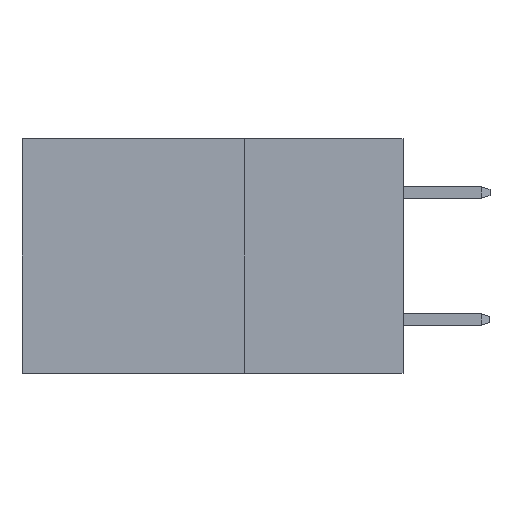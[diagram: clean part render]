
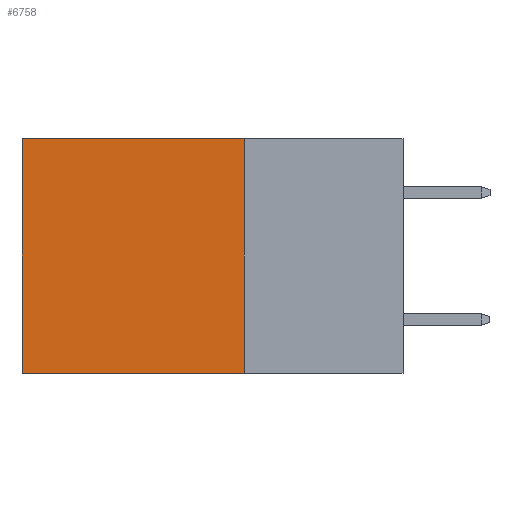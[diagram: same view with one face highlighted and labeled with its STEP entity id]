
A CAD part, left-side view. The second image highlights one B-rep face of the part: STEP entity #6758.
In plain terms, the highlighted planar face has unit normal (-1, 0, 0).
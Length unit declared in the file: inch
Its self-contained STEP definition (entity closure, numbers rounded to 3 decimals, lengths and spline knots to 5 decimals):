
#52 = VERTEX_POINT ( 'NONE', #12738 ) ;
#105 = CARTESIAN_POINT ( 'NONE',  ( 0.2875, 0.6, -0.37 ) ) ;
#437 = ORIENTED_EDGE ( 'NONE', *, *, #8776, .F. ) ;
#654 = DIRECTION ( 'NONE',  ( 0., 0., -1. ) ) ;
#732 = DIRECTION ( 'NONE',  ( 1., 0., 0. ) ) ;
#789 = EDGE_CURVE ( 'NONE', #52, #1972, #9901, .T. ) ;
#849 = PLANE ( 'NONE',  #10266 ) ;
#1972 = VERTEX_POINT ( 'NONE', #105 ) ;
#2182 = VERTEX_POINT ( 'NONE', #2674 ) ;
#2674 = CARTESIAN_POINT ( 'NONE',  ( 0.2875, 0.25, -0.37 ) ) ;
#2708 = ORIENTED_EDGE ( 'NONE', *, *, #7751, .T. ) ;
#2967 = CARTESIAN_POINT ( 'NONE',  ( 0.2875, 0.25, 0. ) ) ;
#4094 = ORIENTED_EDGE ( 'NONE', *, *, #789, .T. ) ;
#4709 = CARTESIAN_POINT ( 'NONE',  ( 0.2875, 0.6, 0. ) ) ;
#4719 = FACE_OUTER_BOUND ( 'NONE', #7755, .T. ) ;
#4855 = CARTESIAN_POINT ( 'NONE',  ( 0.2875, 0.25, 0. ) ) ;
#4874 = LINE ( 'NONE', #2967, #11093 ) ;
#4888 = EDGE_CURVE ( 'NONE', #2182, #1972, #9230, .T. ) ;
#6582 = LINE ( 'NONE', #12035, #8116 ) ;
#6758 = ADVANCED_FACE ( 'NONE', ( #4719 ), #849, .F. ) ;
#7716 = VECTOR ( 'NONE', #654, 39.37008 ) ;
#7751 = EDGE_CURVE ( 'NONE', #9471, #52, #6582, .T. ) ;
#7755 = EDGE_LOOP ( 'NONE', ( #4094, #12394, #437, #2708 ) ) ;
#8116 = VECTOR ( 'NONE', #10898, 39.37008 ) ;
#8776 = EDGE_CURVE ( 'NONE', #9471, #2182, #4874, .T. ) ;
#9230 = LINE ( 'NONE', #12243, #12608 ) ;
#9471 = VERTEX_POINT ( 'NONE', #11818 ) ;
#9901 = LINE ( 'NONE', #4709, #7716 ) ;
#9912 = DIRECTION ( 'NONE',  ( 0., 0., -1. ) ) ;
#10266 = AXIS2_PLACEMENT_3D ( 'NONE', #4855, #732, #9912 ) ;
#10317 = DIRECTION ( 'NONE',  ( 0., 0., -1. ) ) ;
#10898 = DIRECTION ( 'NONE',  ( 0., 1., 0. ) ) ;
#11093 = VECTOR ( 'NONE', #10317, 39.37008 ) ;
#11818 = CARTESIAN_POINT ( 'NONE',  ( 0.2875, 0.25, 0. ) ) ;
#12035 = CARTESIAN_POINT ( 'NONE',  ( 0.2875, 0.25, 0. ) ) ;
#12243 = CARTESIAN_POINT ( 'NONE',  ( 0.2875, 0.25, -0.37 ) ) ;
#12394 = ORIENTED_EDGE ( 'NONE', *, *, #4888, .F. ) ;
#12608 = VECTOR ( 'NONE', #13308, 39.37008 ) ;
#12738 = CARTESIAN_POINT ( 'NONE',  ( 0.2875, 0.6, 0. ) ) ;
#13308 = DIRECTION ( 'NONE',  ( 0., 1., 0. ) ) ;
